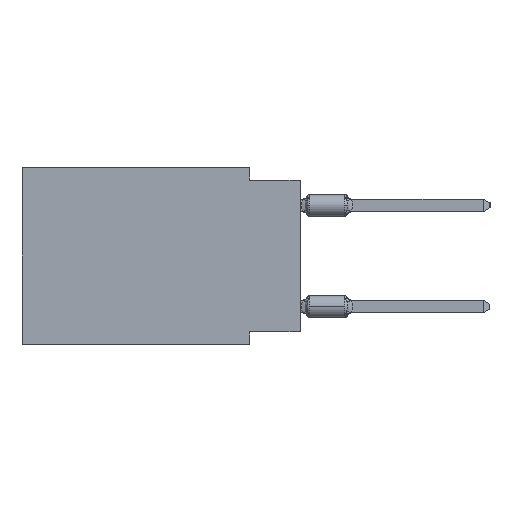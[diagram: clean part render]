
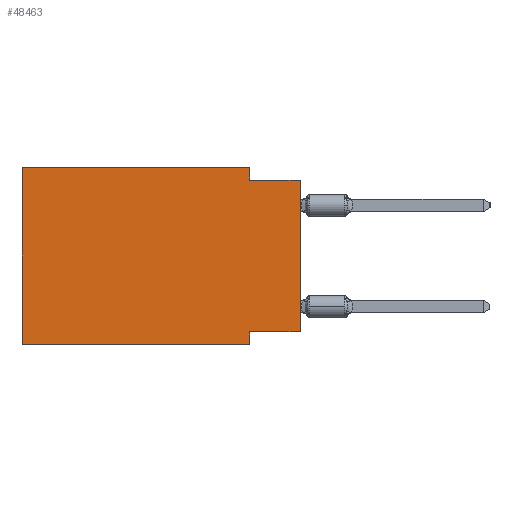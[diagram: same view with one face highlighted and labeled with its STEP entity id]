
A CAD part, left-side view. The second image highlights one B-rep face of the part: STEP entity #48463.
In plain terms, the highlighted planar face has unit normal (-1, 0, 0).
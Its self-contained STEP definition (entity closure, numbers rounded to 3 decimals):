
#656 = LINE ( 'NONE', #47579, #8238 ) ;
#1275 = ORIENTED_EDGE ( 'NONE', *, *, #8446, .F. ) ;
#1931 = DIRECTION ( 'NONE',  ( 0., -1., 0. ) ) ;
#2793 = ORIENTED_EDGE ( 'NONE', *, *, #26551, .F. ) ;
#2918 = DIRECTION ( 'NONE',  ( 0., 0., -1. ) ) ;
#3278 = LINE ( 'NONE', #20360, #21000 ) ;
#3950 = VECTOR ( 'NONE', #35120, 1000. ) ;
#4306 = DIRECTION ( 'NONE',  ( 0., 1., 0. ) ) ;
#4586 = CARTESIAN_POINT ( 'NONE',  ( 0., 13.97, -8.89 ) ) ;
#8017 = EDGE_LOOP ( 'NONE', ( #24062, #1275, #34258, #53762, #44418, #33617, #2793, #48126 ) ) ;
#8118 = CARTESIAN_POINT ( 'NONE',  ( 0., 13.97, 0. ) ) ;
#8238 = VECTOR ( 'NONE', #49655, 1000. ) ;
#8446 = EDGE_CURVE ( 'NONE', #49300, #52050, #31049, .T. ) ;
#10942 = CARTESIAN_POINT ( 'NONE',  ( 0., 0., -8.255 ) ) ;
#11047 = PLANE ( 'NONE',  #21729 ) ;
#12051 = CARTESIAN_POINT ( 'NONE',  ( 0., 13.97, -8.89 ) ) ;
#13534 = CARTESIAN_POINT ( 'NONE',  ( 0., 0., -8.255 ) ) ;
#17871 = VECTOR ( 'NONE', #34102, 1000. ) ;
#18077 = EDGE_CURVE ( 'NONE', #42016, #49300, #22737, .T. ) ;
#18220 = VERTEX_POINT ( 'NONE', #4586 ) ;
#18368 = DIRECTION ( 'NONE',  ( 0., 0., 1. ) ) ;
#18635 = CARTESIAN_POINT ( 'NONE',  ( 0., 13.97, 0. ) ) ;
#20360 = CARTESIAN_POINT ( 'NONE',  ( 0., 13.97, 0. ) ) ;
#20486 = EDGE_CURVE ( 'NONE', #26620, #42016, #3278, .T. ) ;
#21000 = VECTOR ( 'NONE', #37367, 1000. ) ;
#21440 = CARTESIAN_POINT ( 'NONE',  ( 0., 0., -0.635 ) ) ;
#21729 = AXIS2_PLACEMENT_3D ( 'NONE', #40644, #40357, #2918 ) ;
#22737 = LINE ( 'NONE', #35814, #43956 ) ;
#22958 = CARTESIAN_POINT ( 'NONE',  ( 0., 0., -0.635 ) ) ;
#24062 = ORIENTED_EDGE ( 'NONE', *, *, #42237, .T. ) ;
#26551 = EDGE_CURVE ( 'NONE', #43731, #27516, #43489, .T. ) ;
#26620 = VERTEX_POINT ( 'NONE', #8118 ) ;
#27516 = VERTEX_POINT ( 'NONE', #44197 ) ;
#27615 = VERTEX_POINT ( 'NONE', #10942 ) ;
#28294 = EDGE_CURVE ( 'NONE', #18220, #27516, #37199, .T. ) ;
#29296 = CARTESIAN_POINT ( 'NONE',  ( 0., 2.54, -0.635 ) ) ;
#30118 = CARTESIAN_POINT ( 'NONE',  ( 0., 2.54, -8.89 ) ) ;
#31049 = LINE ( 'NONE', #22958, #49669 ) ;
#31919 = DIRECTION ( 'NONE',  ( 0., 0., -1. ) ) ;
#33617 = ORIENTED_EDGE ( 'NONE', *, *, #28294, .T. ) ;
#33659 = CARTESIAN_POINT ( 'NONE',  ( 0., 2.54, 0. ) ) ;
#34102 = DIRECTION ( 'NONE',  ( 0., -1., 0. ) ) ;
#34258 = ORIENTED_EDGE ( 'NONE', *, *, #18077, .F. ) ;
#35120 = DIRECTION ( 'NONE',  ( 0., 0., -1. ) ) ;
#35814 = CARTESIAN_POINT ( 'NONE',  ( 0., 2.54, 0. ) ) ;
#37199 = LINE ( 'NONE', #12051, #17871 ) ;
#37367 = DIRECTION ( 'NONE',  ( 0., -1., 0. ) ) ;
#39560 = LINE ( 'NONE', #18635, #48453 ) ;
#40357 = DIRECTION ( 'NONE',  ( 1., 0., 0. ) ) ;
#40644 = CARTESIAN_POINT ( 'NONE',  ( 0., 13.97, 0. ) ) ;
#41185 = FACE_OUTER_BOUND ( 'NONE', #8017, .T. ) ;
#42016 = VERTEX_POINT ( 'NONE', #33659 ) ;
#42237 = EDGE_CURVE ( 'NONE', #27615, #52050, #656, .T. ) ;
#43489 = LINE ( 'NONE', #30118, #3950 ) ;
#43731 = VERTEX_POINT ( 'NONE', #54959 ) ;
#43956 = VECTOR ( 'NONE', #31919, 1000. ) ;
#44197 = CARTESIAN_POINT ( 'NONE',  ( 0., 2.54, -8.89 ) ) ;
#44418 = ORIENTED_EDGE ( 'NONE', *, *, #53450, .F. ) ;
#47326 = LINE ( 'NONE', #13534, #53798 ) ;
#47579 = CARTESIAN_POINT ( 'NONE',  ( 0., 0., 0. ) ) ;
#48126 = ORIENTED_EDGE ( 'NONE', *, *, #53647, .F. ) ;
#48453 = VECTOR ( 'NONE', #18368, 1000. ) ;
#48463 = ADVANCED_FACE ( 'NONE', ( #41185 ), #11047, .F. ) ;
#49300 = VERTEX_POINT ( 'NONE', #29296 ) ;
#49655 = DIRECTION ( 'NONE',  ( 0., 0., 1. ) ) ;
#49669 = VECTOR ( 'NONE', #1931, 1000. ) ;
#52050 = VERTEX_POINT ( 'NONE', #21440 ) ;
#53450 = EDGE_CURVE ( 'NONE', #18220, #26620, #39560, .T. ) ;
#53647 = EDGE_CURVE ( 'NONE', #27615, #43731, #47326, .T. ) ;
#53762 = ORIENTED_EDGE ( 'NONE', *, *, #20486, .F. ) ;
#53798 = VECTOR ( 'NONE', #4306, 1000. ) ;
#54959 = CARTESIAN_POINT ( 'NONE',  ( 0., 2.54, -8.255 ) ) ;
